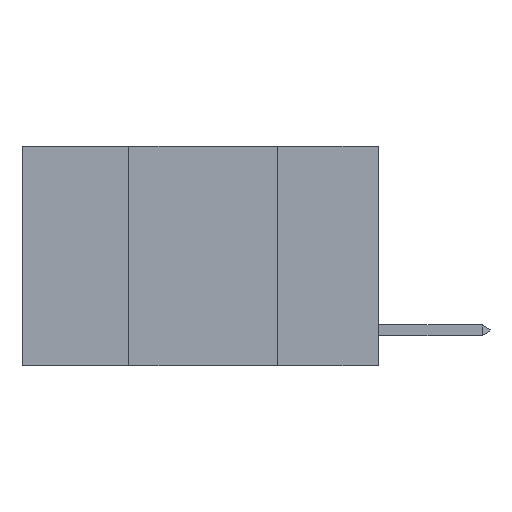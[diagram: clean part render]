
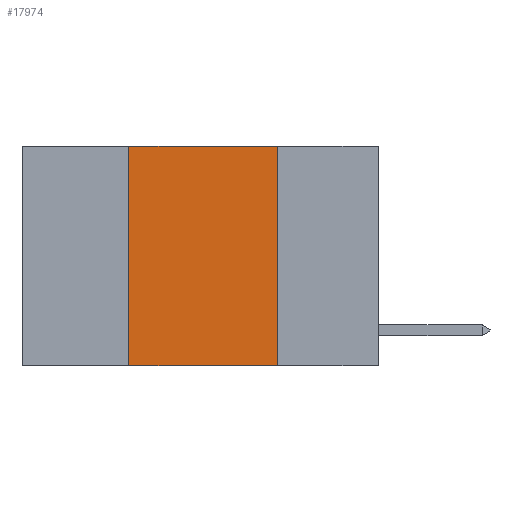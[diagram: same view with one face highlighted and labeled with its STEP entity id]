
A CAD part, left-side view. The second image highlights one B-rep face of the part: STEP entity #17974.
In plain terms, the highlighted planar face has unit normal (-1, 0, 0).
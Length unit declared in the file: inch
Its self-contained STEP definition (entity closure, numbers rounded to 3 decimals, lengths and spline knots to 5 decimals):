
#1179 = LINE ( 'NONE', #8144, #10640 ) ;
#1453 = VECTOR ( 'NONE', #1559, 39.37008 ) ;
#1559 = DIRECTION ( 'NONE',  ( 0., -1., 0. ) ) ;
#2355 = DIRECTION ( 'NONE',  ( 0., 0., -1. ) ) ;
#2384 = ORIENTED_EDGE ( 'NONE', *, *, #18848, .F. ) ;
#4868 = CARTESIAN_POINT ( 'NONE',  ( 0., 0.6, 0. ) ) ;
#5278 = CARTESIAN_POINT ( 'NONE',  ( 0., 0.42, -0.37 ) ) ;
#5737 = VERTEX_POINT ( 'NONE', #13925 ) ;
#5848 = CARTESIAN_POINT ( 'NONE',  ( 0., 0.17, 0. ) ) ;
#6661 = DIRECTION ( 'NONE',  ( 0., 0., -1. ) ) ;
#7175 = LINE ( 'NONE', #19483, #16053 ) ;
#7660 = EDGE_CURVE ( 'NONE', #13019, #14505, #11351, .T. ) ;
#8144 = CARTESIAN_POINT ( 'NONE',  ( 0., 0.6, -0.37 ) ) ;
#8347 = PLANE ( 'NONE',  #20051 ) ;
#9266 = EDGE_LOOP ( 'NONE', ( #13801, #12925, #2384, #12382 ) ) ;
#10640 = VECTOR ( 'NONE', #20453, 39.37008 ) ;
#10918 = LINE ( 'NONE', #13989, #1453 ) ;
#11351 = LINE ( 'NONE', #5848, #15519 ) ;
#12307 = FACE_OUTER_BOUND ( 'NONE', #9266, .T. ) ;
#12382 = ORIENTED_EDGE ( 'NONE', *, *, #17402, .T. ) ;
#12925 = ORIENTED_EDGE ( 'NONE', *, *, #21673, .F. ) ;
#13019 = VERTEX_POINT ( 'NONE', #16393 ) ;
#13801 = ORIENTED_EDGE ( 'NONE', *, *, #7660, .F. ) ;
#13925 = CARTESIAN_POINT ( 'NONE',  ( 0., 0.42, 0. ) ) ;
#13989 = CARTESIAN_POINT ( 'NONE',  ( 0., 0.6, 0. ) ) ;
#14505 = VERTEX_POINT ( 'NONE', #21708 ) ;
#15519 = VECTOR ( 'NONE', #2355, 39.37008 ) ;
#16053 = VECTOR ( 'NONE', #21227, 39.37008 ) ;
#16393 = CARTESIAN_POINT ( 'NONE',  ( 0., 0.17, 0. ) ) ;
#17269 = DIRECTION ( 'NONE',  ( 1., 0., 0. ) ) ;
#17402 = EDGE_CURVE ( 'NONE', #19968, #14505, #1179, .T. ) ;
#17974 = ADVANCED_FACE ( 'NONE', ( #12307 ), #8347, .F. ) ;
#18848 = EDGE_CURVE ( 'NONE', #19968, #5737, #7175, .T. ) ;
#19483 = CARTESIAN_POINT ( 'NONE',  ( 0., 0.42, 0. ) ) ;
#19968 = VERTEX_POINT ( 'NONE', #5278 ) ;
#20051 = AXIS2_PLACEMENT_3D ( 'NONE', #4868, #17269, #6661 ) ;
#20453 = DIRECTION ( 'NONE',  ( 0., -1., 0. ) ) ;
#21227 = DIRECTION ( 'NONE',  ( 0., 0., 1. ) ) ;
#21673 = EDGE_CURVE ( 'NONE', #5737, #13019, #10918, .T. ) ;
#21708 = CARTESIAN_POINT ( 'NONE',  ( 0., 0.17, -0.37 ) ) ;
